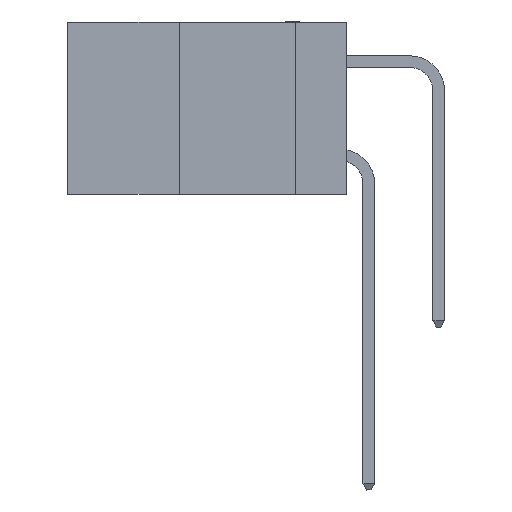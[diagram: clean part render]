
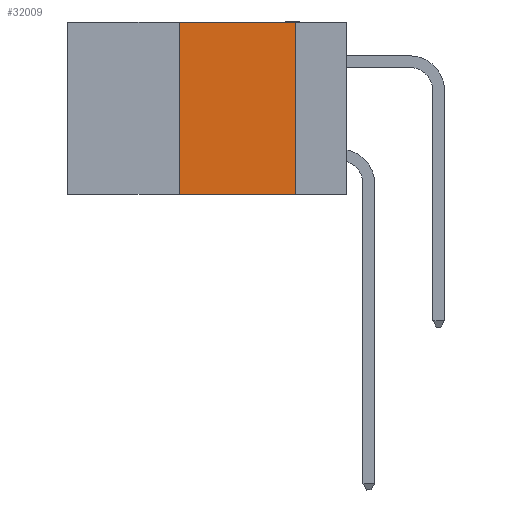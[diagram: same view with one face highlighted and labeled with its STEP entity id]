
A CAD part, left-side view. The second image highlights one B-rep face of the part: STEP entity #32009.
In plain terms, the highlighted planar face has unit normal (-1, 0, 0).
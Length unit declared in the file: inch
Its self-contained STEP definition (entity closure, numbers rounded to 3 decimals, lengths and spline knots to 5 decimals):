
#543 = DIRECTION ( 'NONE',  ( 0., 0., -1. ) ) ;
#876 = CARTESIAN_POINT ( 'NONE',  ( 0., 0.11, -0.37 ) ) ;
#1434 = DIRECTION ( 'NONE',  ( 0., 0., -1. ) ) ;
#1836 = CARTESIAN_POINT ( 'NONE',  ( 0., 0.11, 0. ) ) ;
#2688 = EDGE_LOOP ( 'NONE', ( #8859, #29047, #18669, #16819 ) ) ;
#4078 = LINE ( 'NONE', #11184, #35273 ) ;
#4281 = CARTESIAN_POINT ( 'NONE',  ( 0., 0.11, 0. ) ) ;
#4339 = CARTESIAN_POINT ( 'NONE',  ( 0., 0.36, 0. ) ) ;
#7739 = CARTESIAN_POINT ( 'NONE',  ( 0., 0.36, -0.37 ) ) ;
#8859 = ORIENTED_EDGE ( 'NONE', *, *, #12099, .F. ) ;
#9042 = VERTEX_POINT ( 'NONE', #876 ) ;
#11184 = CARTESIAN_POINT ( 'NONE',  ( 0., 0.6, 0. ) ) ;
#11463 = CARTESIAN_POINT ( 'NONE',  ( 0., 0.36, 0. ) ) ;
#11488 = EDGE_CURVE ( 'NONE', #22412, #9042, #28458, .T. ) ;
#11933 = DIRECTION ( 'NONE',  ( 1., 0., 0. ) ) ;
#12099 = EDGE_CURVE ( 'NONE', #30305, #9042, #30087, .T. ) ;
#15372 = EDGE_CURVE ( 'NONE', #22412, #30091, #25332, .T. ) ;
#16819 = ORIENTED_EDGE ( 'NONE', *, *, #11488, .T. ) ;
#16880 = DIRECTION ( 'NONE',  ( 0., -1., 0. ) ) ;
#16905 = CARTESIAN_POINT ( 'NONE',  ( 0., 0.6, 0. ) ) ;
#17916 = DIRECTION ( 'NONE',  ( 0., -1., 0. ) ) ;
#18087 = VECTOR ( 'NONE', #31707, 39.37008 ) ;
#18669 = ORIENTED_EDGE ( 'NONE', *, *, #15372, .F. ) ;
#19826 = CARTESIAN_POINT ( 'NONE',  ( 0., 0.6, -0.37 ) ) ;
#21548 = AXIS2_PLACEMENT_3D ( 'NONE', #16905, #11933, #543 ) ;
#22412 = VERTEX_POINT ( 'NONE', #7739 ) ;
#23694 = VECTOR ( 'NONE', #1434, 39.37008 ) ;
#25332 = LINE ( 'NONE', #4339, #18087 ) ;
#25343 = FACE_OUTER_BOUND ( 'NONE', #2688, .T. ) ;
#28458 = LINE ( 'NONE', #19826, #34850 ) ;
#29047 = ORIENTED_EDGE ( 'NONE', *, *, #30528, .F. ) ;
#30087 = LINE ( 'NONE', #4281, #23694 ) ;
#30091 = VERTEX_POINT ( 'NONE', #11463 ) ;
#30305 = VERTEX_POINT ( 'NONE', #1836 ) ;
#30528 = EDGE_CURVE ( 'NONE', #30091, #30305, #4078, .T. ) ;
#31707 = DIRECTION ( 'NONE',  ( 0., 0., 1. ) ) ;
#32009 = ADVANCED_FACE ( 'NONE', ( #25343 ), #33285, .F. ) ;
#33285 = PLANE ( 'NONE',  #21548 ) ;
#34850 = VECTOR ( 'NONE', #17916, 39.37008 ) ;
#35273 = VECTOR ( 'NONE', #16880, 39.37008 ) ;
